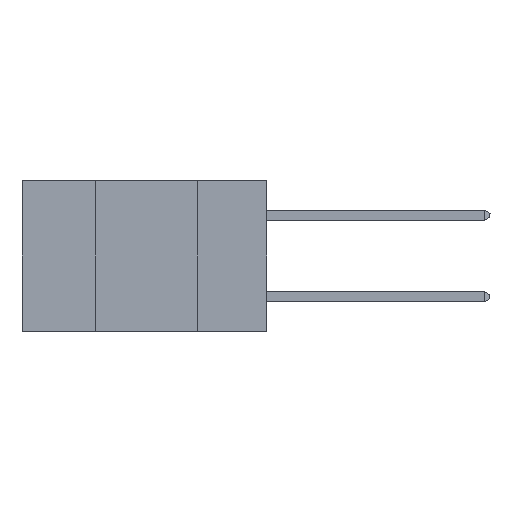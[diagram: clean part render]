
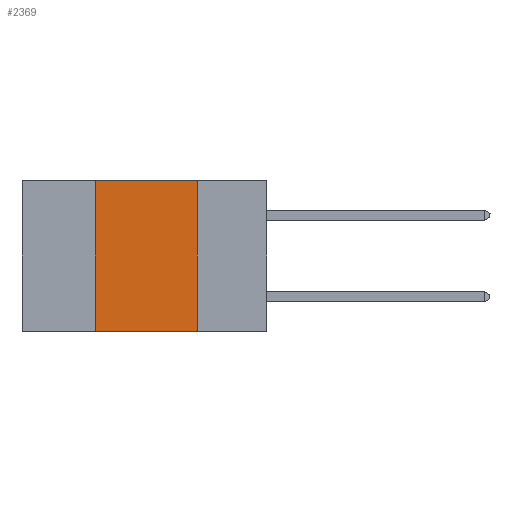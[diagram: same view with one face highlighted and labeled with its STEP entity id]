
A CAD part, left-side view. The second image highlights one B-rep face of the part: STEP entity #2369.
In plain terms, the highlighted planar face has unit normal (-1, 0, 0).
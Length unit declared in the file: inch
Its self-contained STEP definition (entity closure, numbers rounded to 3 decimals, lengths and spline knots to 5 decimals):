
#1216 = CARTESIAN_POINT ( 'NONE',  ( 0., 0.6, 0. ) ) ;
#1229 = VECTOR ( 'NONE', #4892, 39.37008 ) ;
#2169 = LINE ( 'NONE', #19406, #12770 ) ;
#2369 = ADVANCED_FACE ( 'NONE', ( #22027 ), #22161, .F. ) ;
#2967 = DIRECTION ( 'NONE',  ( 1., 0., 0. ) ) ;
#3734 = LINE ( 'NONE', #1216, #10317 ) ;
#4348 = VERTEX_POINT ( 'NONE', #14348 ) ;
#4892 = DIRECTION ( 'NONE',  ( 0., 0., 1. ) ) ;
#5540 = CARTESIAN_POINT ( 'NONE',  ( 0., 0.42, -0.37 ) ) ;
#5705 = LINE ( 'NONE', #22165, #24732 ) ;
#6337 = EDGE_LOOP ( 'NONE', ( #21951, #18856, #16150, #25004 ) ) ;
#7150 = CARTESIAN_POINT ( 'NONE',  ( 0., 0.6, 0. ) ) ;
#7673 = EDGE_CURVE ( 'NONE', #24415, #10910, #15073, .T. ) ;
#8098 = CARTESIAN_POINT ( 'NONE',  ( 0., 0.17, -0.37 ) ) ;
#10039 = EDGE_CURVE ( 'NONE', #10910, #4348, #3734, .T. ) ;
#10317 = VECTOR ( 'NONE', #20556, 39.37008 ) ;
#10910 = VERTEX_POINT ( 'NONE', #12685 ) ;
#11102 = EDGE_CURVE ( 'NONE', #24415, #22563, #5705, .T. ) ;
#12685 = CARTESIAN_POINT ( 'NONE',  ( 0., 0.42, 0. ) ) ;
#12770 = VECTOR ( 'NONE', #17159, 39.37008 ) ;
#13479 = EDGE_CURVE ( 'NONE', #4348, #22563, #2169, .T. ) ;
#14275 = DIRECTION ( 'NONE',  ( 0., -1., 0. ) ) ;
#14348 = CARTESIAN_POINT ( 'NONE',  ( 0., 0.17, 0. ) ) ;
#14763 = AXIS2_PLACEMENT_3D ( 'NONE', #7150, #2967, #22296 ) ;
#15073 = LINE ( 'NONE', #22135, #1229 ) ;
#16150 = ORIENTED_EDGE ( 'NONE', *, *, #7673, .F. ) ;
#17159 = DIRECTION ( 'NONE',  ( 0., 0., -1. ) ) ;
#18856 = ORIENTED_EDGE ( 'NONE', *, *, #10039, .F. ) ;
#19406 = CARTESIAN_POINT ( 'NONE',  ( 0., 0.17, 0. ) ) ;
#20556 = DIRECTION ( 'NONE',  ( 0., -1., 0. ) ) ;
#21951 = ORIENTED_EDGE ( 'NONE', *, *, #13479, .F. ) ;
#22027 = FACE_OUTER_BOUND ( 'NONE', #6337, .T. ) ;
#22135 = CARTESIAN_POINT ( 'NONE',  ( 0., 0.42, 0. ) ) ;
#22161 = PLANE ( 'NONE',  #14763 ) ;
#22165 = CARTESIAN_POINT ( 'NONE',  ( 0., 0.6, -0.37 ) ) ;
#22296 = DIRECTION ( 'NONE',  ( 0., 0., -1. ) ) ;
#22563 = VERTEX_POINT ( 'NONE', #8098 ) ;
#24415 = VERTEX_POINT ( 'NONE', #5540 ) ;
#24732 = VECTOR ( 'NONE', #14275, 39.37008 ) ;
#25004 = ORIENTED_EDGE ( 'NONE', *, *, #11102, .T. ) ;
